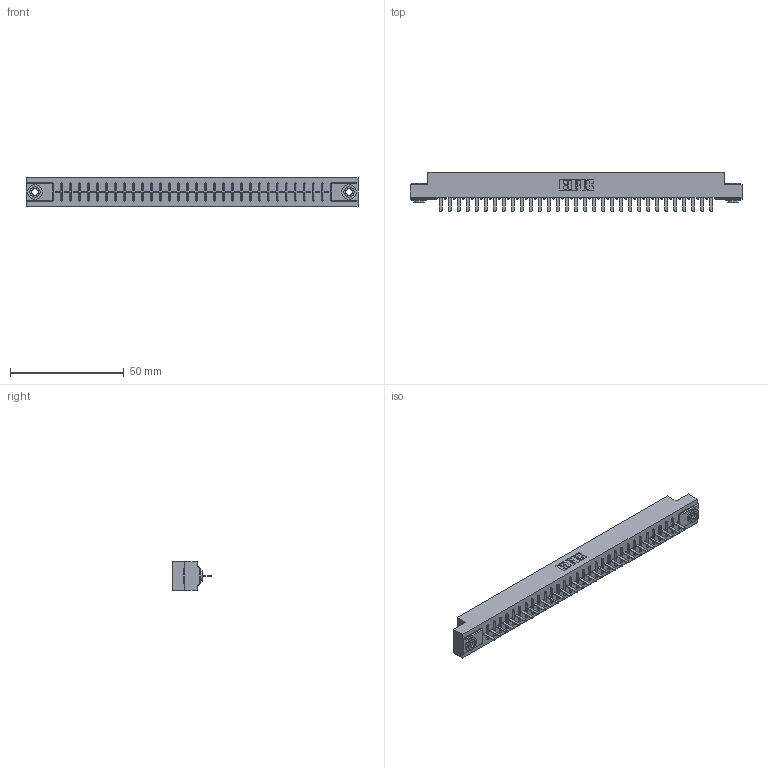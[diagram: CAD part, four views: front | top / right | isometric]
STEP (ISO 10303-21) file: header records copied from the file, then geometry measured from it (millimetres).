
FILE_DESCRIPTION (( 'STEP AP203' ), '1' );
FILE_NAME ('306-031-420-103.STEP', '2020-09-22T01:42:04', ( '' ), ( '' ), 'SwSTEP 2.0', 'SolidWorks 2020', '' );
FILE_SCHEMA (( 'CONFIG_CONTROL_DESIGN' ));
Length unit declared in the file: inch
Products named in the file (4): 306 Part_.156 Dia; 306-031-420-103; 345-250-002_345-250-002-102; 306-290-001_120
Assembly tree (34 placements, depth 2):
  306-031-420-103
    306 Part_.156 Dia
    306-290-001_120  x31
    345-250-002_345-250-002-102  x2
Bounding box: 145.85 x 17.12 x 12.7 mm (x, y, z)
Volume: 16031.8 mm3; surface area: 16608.3 mm2
Topology: 34 solids, 34 shells, 2338 faces, 6535 edges, 4186 vertices
Faces by surface type: plane 1549, cylinder 657, sphere 124, cone 8
Entity records: 31355 total; most frequent: CARTESIAN_POINT 5241, ORIENTED_EDGE 5186, DIRECTION 5183, EDGE_CURVE 2593, LINE 2015, VECTOR 2015, VERTEX_POINT 1642, AXIS2_PLACEMENT_3D 1584
